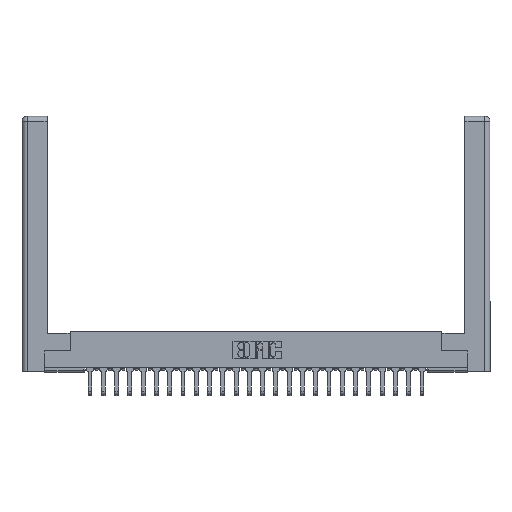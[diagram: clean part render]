
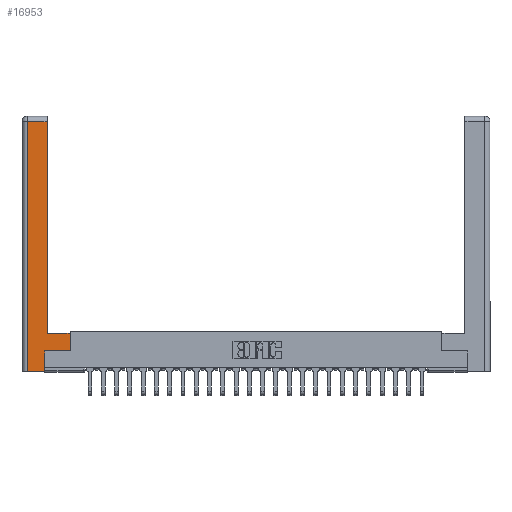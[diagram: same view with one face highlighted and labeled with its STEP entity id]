
A CAD part, top view. The second image highlights one B-rep face of the part: STEP entity #16953.
In plain terms, the highlighted planar face has unit normal (0, 0, 1).
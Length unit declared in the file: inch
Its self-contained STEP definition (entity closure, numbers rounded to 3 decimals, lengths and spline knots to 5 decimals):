
#204 = VERTEX_POINT ( 'NONE', #14951 ) ;
#442 = LINE ( 'NONE', #20404, #11886 ) ;
#582 = VECTOR ( 'NONE', #20364, 39.37008 ) ;
#1126 = EDGE_LOOP ( 'NONE', ( #27841, #25247, #16341, #22972, #14402, #6476, #12518, #26220 ) ) ;
#3005 = DIRECTION ( 'NONE',  ( 1., 0., 0. ) ) ;
#3437 = DIRECTION ( 'NONE',  ( 0., 1., 0. ) ) ;
#4082 = VECTOR ( 'NONE', #3437, 39.37008 ) ;
#5036 = CARTESIAN_POINT ( 'NONE',  ( 0.295, 0.45, 0. ) ) ;
#5842 = VERTEX_POINT ( 'NONE', #27515 ) ;
#6476 = ORIENTED_EDGE ( 'NONE', *, *, #9567, .T. ) ;
#7158 = VERTEX_POINT ( 'NONE', #18613 ) ;
#7437 = EDGE_CURVE ( 'NONE', #204, #7158, #24508, .T. ) ;
#8209 = LINE ( 'NONE', #21842, #17844 ) ;
#9567 = EDGE_CURVE ( 'NONE', #23848, #9929, #24307, .T. ) ;
#9858 = LINE ( 'NONE', #27767, #26237 ) ;
#9929 = VERTEX_POINT ( 'NONE', #16582 ) ;
#10042 = VERTEX_POINT ( 'NONE', #26920 ) ;
#10295 = FACE_OUTER_BOUND ( 'NONE', #1126, .T. ) ;
#10367 = CARTESIAN_POINT ( 'NONE',  ( 0.265, 0., 0. ) ) ;
#10685 = DIRECTION ( 'NONE',  ( 1., 0., 0. ) ) ;
#11886 = VECTOR ( 'NONE', #18344, 39.37008 ) ;
#11954 = EDGE_CURVE ( 'NONE', #10042, #29013, #9858, .T. ) ;
#12518 = ORIENTED_EDGE ( 'NONE', *, *, #20793, .T. ) ;
#13068 = EDGE_CURVE ( 'NONE', #29013, #16266, #19413, .T. ) ;
#13273 = VECTOR ( 'NONE', #3005, 39.37008 ) ;
#13787 = VECTOR ( 'NONE', #17570, 39.37008 ) ;
#13898 = VECTOR ( 'NONE', #10685, 39.37008 ) ;
#14402 = ORIENTED_EDGE ( 'NONE', *, *, #22233, .T. ) ;
#14951 = CARTESIAN_POINT ( 'NONE',  ( 0.0615, 2.94, 0. ) ) ;
#15329 = DIRECTION ( 'NONE',  ( -1., 0., 0. ) ) ;
#15497 = LINE ( 'NONE', #27168, #582 ) ;
#15914 = EDGE_CURVE ( 'NONE', #16266, #204, #8209, .T. ) ;
#16266 = VERTEX_POINT ( 'NONE', #17626 ) ;
#16341 = ORIENTED_EDGE ( 'NONE', *, *, #7437, .T. ) ;
#16582 = CARTESIAN_POINT ( 'NONE',  ( 0.565, 0.245, 0. ) ) ;
#16953 = ADVANCED_FACE ( 'NONE', ( #10295 ), #23761, .F. ) ;
#17570 = DIRECTION ( 'NONE',  ( 0., -1., 0. ) ) ;
#17626 = CARTESIAN_POINT ( 'NONE',  ( 0.295, 2.94, 0. ) ) ;
#17844 = VECTOR ( 'NONE', #15329, 39.37008 ) ;
#18344 = DIRECTION ( 'NONE',  ( 0., 1., 0. ) ) ;
#18613 = CARTESIAN_POINT ( 'NONE',  ( 0.0615, 0., 0. ) ) ;
#19113 = CARTESIAN_POINT ( 'NONE',  ( 0.265, 0.245, 0. ) ) ;
#19194 = DIRECTION ( 'NONE',  ( 0., 0., -1. ) ) ;
#19413 = LINE ( 'NONE', #23694, #4082 ) ;
#20013 = CARTESIAN_POINT ( 'NONE',  ( 0.565, 0.245, 0. ) ) ;
#20277 = EDGE_CURVE ( 'NONE', #7158, #5842, #21486, .T. ) ;
#20364 = DIRECTION ( 'NONE',  ( 0., 1., 0. ) ) ;
#20404 = CARTESIAN_POINT ( 'NONE',  ( 0.265, 0.245, 0. ) ) ;
#20793 = EDGE_CURVE ( 'NONE', #9929, #10042, #15497, .T. ) ;
#20976 = DIRECTION ( 'NONE',  ( -1., 0., 0. ) ) ;
#21398 = CARTESIAN_POINT ( 'NONE',  ( 0., 0., 0. ) ) ;
#21486 = LINE ( 'NONE', #10367, #13273 ) ;
#21842 = CARTESIAN_POINT ( 'NONE',  ( 0.0615, 2.94, 0. ) ) ;
#22233 = EDGE_CURVE ( 'NONE', #5842, #23848, #442, .T. ) ;
#22604 = AXIS2_PLACEMENT_3D ( 'NONE', #21398, #19194, #28204 ) ;
#22972 = ORIENTED_EDGE ( 'NONE', *, *, #20277, .T. ) ;
#23694 = CARTESIAN_POINT ( 'NONE',  ( 0.295, 3., 0. ) ) ;
#23761 = PLANE ( 'NONE',  #22604 ) ;
#23848 = VERTEX_POINT ( 'NONE', #19113 ) ;
#24307 = LINE ( 'NONE', #20013, #13898 ) ;
#24508 = LINE ( 'NONE', #26877, #13787 ) ;
#25247 = ORIENTED_EDGE ( 'NONE', *, *, #15914, .T. ) ;
#26220 = ORIENTED_EDGE ( 'NONE', *, *, #11954, .T. ) ;
#26237 = VECTOR ( 'NONE', #20976, 39.37008 ) ;
#26877 = CARTESIAN_POINT ( 'NONE',  ( 0.0615, 0., 0. ) ) ;
#26920 = CARTESIAN_POINT ( 'NONE',  ( 0.565, 0.45, 0. ) ) ;
#27168 = CARTESIAN_POINT ( 'NONE',  ( 0.565, 0.45, 0. ) ) ;
#27515 = CARTESIAN_POINT ( 'NONE',  ( 0.265, 0., 0. ) ) ;
#27767 = CARTESIAN_POINT ( 'NONE',  ( 0.295, 0.45, 0. ) ) ;
#27841 = ORIENTED_EDGE ( 'NONE', *, *, #13068, .T. ) ;
#28204 = DIRECTION ( 'NONE',  ( -1., 0., 0. ) ) ;
#29013 = VERTEX_POINT ( 'NONE', #5036 ) ;
